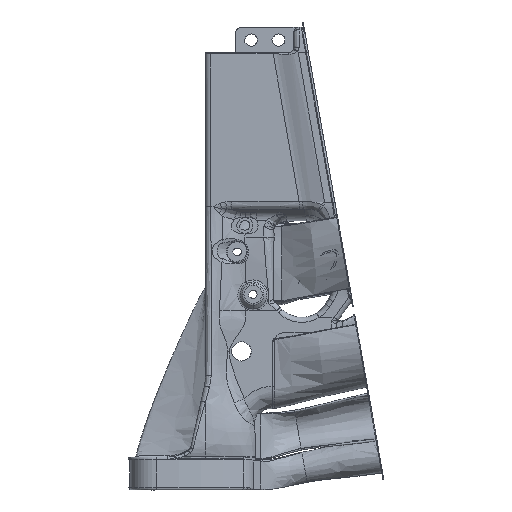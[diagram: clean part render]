
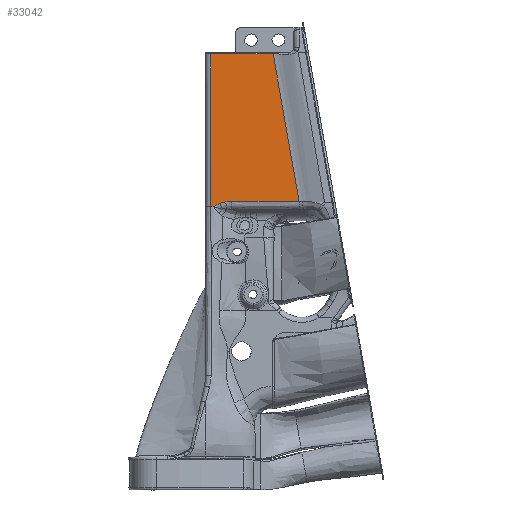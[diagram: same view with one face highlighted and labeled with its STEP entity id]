
A CAD part, left-side view. The second image highlights one B-rep face of the part: STEP entity #33042.
In plain terms, the highlighted planar face has unit normal (-1, 0, 0).
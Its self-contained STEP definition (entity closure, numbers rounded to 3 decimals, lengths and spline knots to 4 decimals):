
#6 = VERTEX_POINT ( 'NONE', #227667 ) ;
#375 = AXIS2_PLACEMENT_3D ( 'NONE', #112674, #20860, #202195 ) ;
#712 = ORIENTED_EDGE ( 'NONE', *, *, #190291, .T. ) ;
#1831 = FACE_OUTER_BOUND ( 'NONE', #233306, .T. ) ;
#3670 = CARTESIAN_POINT ( 'NONE',  ( -0.78, -0.1, 6.615 ) ) ;
#4499 = ORIENTED_EDGE ( 'NONE', *, *, #189318, .T. ) ;
#10991 = EDGE_CURVE ( 'NONE', #38509, #40102, #205928, .T. ) ;
#12209 = CARTESIAN_POINT ( 'NONE',  ( -0.78, -1.8484, 3.7058 ) ) ;
#13493 = CARTESIAN_POINT ( 'NONE',  ( -0.78, -0.2534, 3.6501 ) ) ;
#14082 = VECTOR ( 'NONE', #134483, 39.3701 ) ;
#14643 = CARTESIAN_POINT ( 'NONE',  ( -0.78, -0.2494, 3.6478 ) ) ;
#17967 = CARTESIAN_POINT ( 'NONE',  ( -0.78, -1.3354, 6.615 ) ) ;
#19817 = CARTESIAN_POINT ( 'NONE',  ( -0.78, -0.1, 3.6009 ) ) ;
#20716 = VERTEX_POINT ( 'NONE', #32189 ) ;
#20860 = DIRECTION ( 'NONE',  ( -1., 0., 0. ) ) ;
#20990 = CARTESIAN_POINT ( 'NONE',  ( -0.78, -0.1084, 3.6011 ) ) ;
#21227 = CARTESIAN_POINT ( 'NONE',  ( -0.78, -1.9593, 3.0767 ) ) ;
#30216 = CARTESIAN_POINT ( 'NONE',  ( -0.78, -0.5213, 3.7058 ) ) ;
#31394 = CARTESIAN_POINT ( 'NONE',  ( -0.78, -0.24, 3.6423 ) ) ;
#32189 = CARTESIAN_POINT ( 'NONE',  ( -0.78, -0.2895, 3.6679 ) ) ;
#32425 = ORIENTED_EDGE ( 'NONE', *, *, #155686, .T. ) ;
#32564 = CARTESIAN_POINT ( 'NONE',  ( -0.78, -0.256, 3.6517 ) ) ;
#33042 = ADVANCED_FACE ( 'NONE', ( #1831 ), #73375, .T. ) ;
#38509 = VERTEX_POINT ( 'NONE', #113130 ) ;
#40102 = VERTEX_POINT ( 'NONE', #192219 ) ;
#41042 = CARTESIAN_POINT ( 'NONE',  ( -0.78, -0.5213, 3.7058 ) ) ;
#54446 = CARTESIAN_POINT ( 'NONE',  ( -0.78, -0.1495, 3.6024 ) ) ;
#62350 = CARTESIAN_POINT ( 'NONE',  ( -0.78, -0.5213, 3.7058 ) ) ;
#63794 = CARTESIAN_POINT ( 'NONE',  ( -0.78, -0.3587, 3.6881 ) ) ;
#63941 = EDGE_CURVE ( 'NONE', #68406, #6, #69945, .T. ) ;
#65950 = EDGE_CURVE ( 'NONE', #207586, #68406, #143467, .T. ) ;
#67178 = CARTESIAN_POINT ( 'NONE',  ( -0.78, -0.1638, 3.6064 ) ) ;
#68406 = VERTEX_POINT ( 'NONE', #41042 ) ;
#69945 = B_SPLINE_CURVE_WITH_KNOTS ( 'NONE', 3,
 ( #62350, #137480, #117198, #12209 ),
 .UNSPECIFIED., .F., .F.,
 ( 4, 4 ),
 ( 0.0266, 0.0603 ),
 .UNSPECIFIED. ) ;
#73375 = PLANE ( 'NONE',  #375 ) ;
#76401 = CARTESIAN_POINT ( 'NONE',  ( -0.78, -0.1, 5.6103 ) ) ;
#86239 = CARTESIAN_POINT ( 'NONE',  ( -0.78, -0.2574, 3.6526 ) ) ;
#110446 = CARTESIAN_POINT ( 'NONE',  ( -0.78, -0.1295, 3.6017 ) ) ;
#112674 = CARTESIAN_POINT ( 'NONE',  ( -0.78, -2.8963, 6.64 ) ) ;
#112808 = CARTESIAN_POINT ( 'NONE',  ( -0.78, -0.1505, 3.6025 ) ) ;
#113130 = CARTESIAN_POINT ( 'NONE',  ( -0.78, -0.1, 6.615 ) ) ;
#113323 = ORIENTED_EDGE ( 'NONE', *, *, #63941, .T. ) ;
#117198 = CARTESIAN_POINT ( 'NONE',  ( -0.78, -1.406, 3.7058 ) ) ;
#126612 = DIRECTION ( 'NONE',  ( 0., 1., 0. ) ) ;
#126764 = CARTESIAN_POINT ( 'NONE',  ( -0.78, -0.2051, 3.6234 ) ) ;
#127238 = CARTESIAN_POINT ( 'NONE',  ( -0.78, -0.15, 3.6023 ) ) ;
#134483 = DIRECTION ( 'NONE',  ( 0., 0.174, 0.985 ) ) ;
#135877 = VERTEX_POINT ( 'NONE', #196131 ) ;
#136514 = ORIENTED_EDGE ( 'NONE', *, *, #155897, .T. ) ;
#137480 = CARTESIAN_POINT ( 'NONE',  ( -0.78, -0.9637, 3.7058 ) ) ;
#139828 = LINE ( 'NONE', #143366, #166525 ) ;
#139974 = CARTESIAN_POINT ( 'NONE',  ( -0.78, -0.2239, 3.6331 ) ) ;
#139986 = CARTESIAN_POINT ( 'NONE',  ( -0.78, -0.3956, 3.6953 ) ) ;
#142129 = ORIENTED_EDGE ( 'NONE', *, *, #222444, .T. ) ;
#142330 = CARTESIAN_POINT ( 'NONE',  ( -0.78, -0.2212, 3.6317 ) ) ;
#143366 = CARTESIAN_POINT ( 'NONE',  ( -0.78, -0.1, 6.615 ) ) ;
#143467 = B_SPLINE_CURVE_WITH_KNOTS ( 'NONE', 3,
 ( #139986, #180228, #192489, #30216 ),
 .UNSPECIFIED., .F., .F.,
 ( 4, 4 ),
 ( 0., 1. ),
 .UNSPECIFIED. ) ;
#143513 = CARTESIAN_POINT ( 'NONE',  ( -0.78, -0.1832, 3.6134 ) ) ;
#143971 = CARTESIAN_POINT ( 'NONE',  ( -0.78, -0.14, 3.6021 ) ) ;
#145143 = CARTESIAN_POINT ( 'NONE',  ( -0.78, -0.1337, 3.6019 ) ) ;
#146328 = CARTESIAN_POINT ( 'NONE',  ( -0.78, -0.1484, 3.6023 ) ) ;
#147492 = CARTESIAN_POINT ( 'NONE',  ( -0.78, -0.1432, 3.6022 ) ) ;
#149229 = CARTESIAN_POINT ( 'NONE',  ( -0.78, -0.1, 4.6056 ) ) ;
#151246 = ORIENTED_EDGE ( 'NONE', *, *, #10991, .T. ) ;
#155686 = EDGE_CURVE ( 'NONE', #40102, #135877, #218149, .T. ) ;
#155897 = EDGE_CURVE ( 'NONE', #20716, #207586, #212223, .T. ) ;
#157889 = CARTESIAN_POINT ( 'NONE',  ( -0.78, -0.1505, 3.6025 ) ) ;
#158860 = VERTEX_POINT ( 'NONE', #17967 ) ;
#159046 = CARTESIAN_POINT ( 'NONE',  ( -0.78, -0.269, 3.6595 ) ) ;
#162581 = CARTESIAN_POINT ( 'NONE',  ( -0.78, -0.2159, 3.6288 ) ) ;
#163039 = CARTESIAN_POINT ( 'NONE',  ( -0.78, -0.1168, 3.6014 ) ) ;
#166525 = VECTOR ( 'NONE', #126612, 39.3701 ) ;
#175377 = B_SPLINE_CURVE_WITH_KNOTS ( 'NONE', 3,
 ( #157889, #67178, #143513, #126764, #162581, #142330, #139974, #179303, #215066, #212718, #176970, #31394, #14643, #13493, #32564, #86239, #159046, #235338, #213887 ),
 .UNSPECIFIED., .F., .F.,
 ( 4, 1, 1, 1, 1, 1, 2, 2, 1, 1, 2, 2, 4 ),
 ( 0., 0.25, 0.375, 0.4375, 0.4687, 0.4844, 0.4922, 0.5, 0.625, 0.6875, 0.7187, 0.75, 1. ),
 .UNSPECIFIED. ) ;
#176970 = CARTESIAN_POINT ( 'NONE',  ( -0.78, -0.2319, 3.6377 ) ) ;
#179303 = CARTESIAN_POINT ( 'NONE',  ( -0.78, -0.225, 3.6338 ) ) ;
#180228 = CARTESIAN_POINT ( 'NONE',  ( -0.78, -0.4315, 3.7023 ) ) ;
#188210 = LINE ( 'NONE', #21227, #14082 ) ;
#189318 = EDGE_CURVE ( 'NONE', #6, #158860, #188210, .T. ) ;
#190291 = EDGE_CURVE ( 'NONE', #158860, #38509, #139828, .T. ) ;
#192219 = CARTESIAN_POINT ( 'NONE',  ( -0.78, -0.1, 3.6009 ) ) ;
#192489 = CARTESIAN_POINT ( 'NONE',  ( -0.78, -0.4734, 3.7058 ) ) ;
#196131 = CARTESIAN_POINT ( 'NONE',  ( -0.78, -0.1505, 3.6025 ) ) ;
#202195 = DIRECTION ( 'NONE',  ( 0., 0., 1. ) ) ;
#205928 = B_SPLINE_CURVE_WITH_KNOTS ( 'NONE', 3,
 ( #3670, #76401, #149229, #221975 ),
 .UNSPECIFIED., .F., .F.,
 ( 4, 4 ),
 ( -0.1831, -0.1066 ),
 .UNSPECIFIED. ) ;
#207008 = CARTESIAN_POINT ( 'NONE',  ( -0.78, -0.3233, 3.679 ) ) ;
#207586 = VERTEX_POINT ( 'NONE', #221854 ) ;
#209342 = CARTESIAN_POINT ( 'NONE',  ( -0.78, -0.3956, 3.6953 ) ) ;
#212223 = B_SPLINE_CURVE_WITH_KNOTS ( 'NONE', 3,
 ( #224884, #207008, #63794, #209342 ),
 .UNSPECIFIED., .F., .F.,
 ( 4, 4 ),
 ( 0., 1. ),
 .UNSPECIFIED. ) ;
#212718 = CARTESIAN_POINT ( 'NONE',  ( -0.78, -0.2262, 3.6344 ) ) ;
#213887 = CARTESIAN_POINT ( 'NONE',  ( -0.78, -0.2895, 3.6679 ) ) ;
#215066 = CARTESIAN_POINT ( 'NONE',  ( -0.78, -0.2258, 3.6342 ) ) ;
#217889 = CARTESIAN_POINT ( 'NONE',  ( -0.78, -0.1468, 3.6023 ) ) ;
#218149 = B_SPLINE_CURVE_WITH_KNOTS ( 'NONE', 3,
 ( #19817, #20990, #163039, #110446, #145143, #143971, #147492, #217889, #146328, #54446, #127238, #112808 ),
 .UNSPECIFIED., .F., .F.,
 ( 4, 2, 2, 1, 1, 2, 4 ),
 ( 0.0024, 0.0031, 0.0034, 0.0035, 0.0036, 0.0037, 0.0037 ),
 .UNSPECIFIED. ) ;
#221854 = CARTESIAN_POINT ( 'NONE',  ( -0.78, -0.3956, 3.6953 ) ) ;
#221975 = CARTESIAN_POINT ( 'NONE',  ( -0.78, -0.1, 3.6009 ) ) ;
#222444 = EDGE_CURVE ( 'NONE', #135877, #20716, #175377, .T. ) ;
#224884 = CARTESIAN_POINT ( 'NONE',  ( -0.78, -0.2895, 3.6679 ) ) ;
#226227 = ORIENTED_EDGE ( 'NONE', *, *, #65950, .T. ) ;
#227667 = CARTESIAN_POINT ( 'NONE',  ( -0.78, -1.8484, 3.7058 ) ) ;
#233306 = EDGE_LOOP ( 'NONE', ( #4499, #712, #151246, #32425, #142129, #136514, #226227, #113323 ) ) ;
#235338 = CARTESIAN_POINT ( 'NONE',  ( -0.78, -0.2793, 3.6644 ) ) ;
